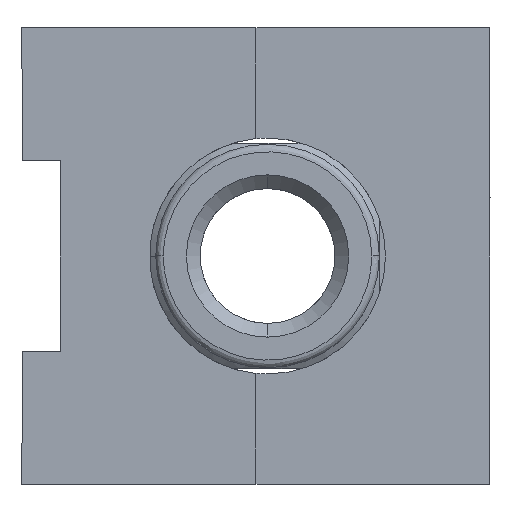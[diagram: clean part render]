
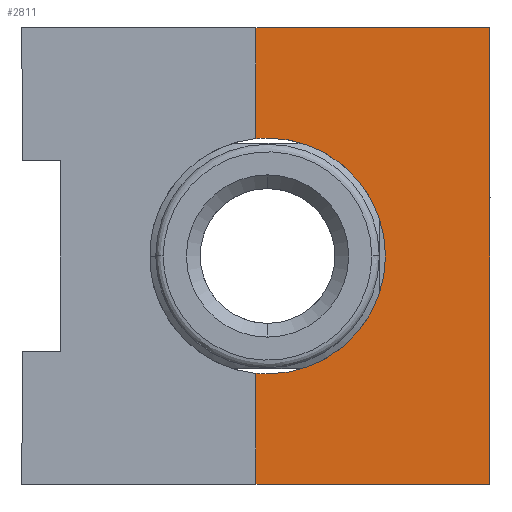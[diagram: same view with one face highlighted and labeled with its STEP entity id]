
A CAD part, left-side view. The second image highlights one B-rep face of the part: STEP entity #2811.
In plain terms, the highlighted planar face has unit normal (-1, 0, 0).
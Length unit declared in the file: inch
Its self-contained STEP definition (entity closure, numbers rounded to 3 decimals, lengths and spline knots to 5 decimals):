
#186 = DIRECTION ( 'NONE',  ( 1., 0., 0. ) ) ;
#281 = CARTESIAN_POINT ( 'NONE',  ( 1.98961, -0.28456, -0.6 ) ) ;
#456 = CIRCLE ( 'NONE', #14050, 0.31 ) ;
#748 = CARTESIAN_POINT ( 'NONE',  ( 1.98961, 0.33044, 0.6 ) ) ;
#859 = ORIENTED_EDGE ( 'NONE', *, *, #3745, .T. ) ;
#975 = CARTESIAN_POINT ( 'NONE',  ( 1.98961, -0.28456, 0.6 ) ) ;
#1020 = CARTESIAN_POINT ( 'NONE',  ( 1.98961, -0.31496, 0. ) ) ;
#1428 = DIRECTION ( 'NONE',  ( 0., 0., -1. ) ) ;
#1697 = VERTEX_POINT ( 'NONE', #14794 ) ;
#1882 = AXIS2_PLACEMENT_3D ( 'NONE', #8262, #4012, #5552 ) ;
#2111 = ORIENTED_EDGE ( 'NONE', *, *, #13435, .T. ) ;
#2472 = VERTEX_POINT ( 'NONE', #7377 ) ;
#2811 = ADVANCED_FACE ( 'NONE', ( #13321 ), #7819, .F. ) ;
#3658 = DIRECTION ( 'NONE',  ( 0., 1., 0. ) ) ;
#3745 = EDGE_CURVE ( 'NONE', #12427, #18177, #10201, .T. ) ;
#4012 = DIRECTION ( 'NONE',  ( 1., 0., 0. ) ) ;
#4221 = LINE ( 'NONE', #975, #6164 ) ;
#4526 = EDGE_CURVE ( 'NONE', #1697, #12427, #4221, .T. ) ;
#4726 = CARTESIAN_POINT ( 'NONE',  ( 1.98961, -0.28456, 0.6 ) ) ;
#5187 = LINE ( 'NONE', #15519, #13426 ) ;
#5552 = DIRECTION ( 'NONE',  ( 0., 0., -1. ) ) ;
#5729 = EDGE_CURVE ( 'NONE', #18177, #12259, #9547, .T. ) ;
#6164 = VECTOR ( 'NONE', #17194, 39.37008 ) ;
#6167 = LINE ( 'NONE', #4726, #6220 ) ;
#6220 = VECTOR ( 'NONE', #14677, 39.37008 ) ;
#7377 = CARTESIAN_POINT ( 'NONE',  ( 1.98961, -0.28456, -0.30851 ) ) ;
#7590 = VECTOR ( 'NONE', #13576, 39.37008 ) ;
#7753 = CARTESIAN_POINT ( 'NONE',  ( 1.98961, -0.31496, 0.31 ) ) ;
#7819 = PLANE ( 'NONE',  #16041 ) ;
#8262 = CARTESIAN_POINT ( 'NONE',  ( 1.98961, -0.31496, 0. ) ) ;
#8572 = CARTESIAN_POINT ( 'NONE',  ( 1.98961, -0.31496, 0. ) ) ;
#8662 = DIRECTION ( 'NONE',  ( 1., 0., 0. ) ) ;
#9135 = CARTESIAN_POINT ( 'NONE',  ( 1.98961, -0.89956, 0.6 ) ) ;
#9434 = DIRECTION ( 'NONE',  ( 0., 0., -1. ) ) ;
#9542 = LINE ( 'NONE', #748, #13119 ) ;
#9547 = CIRCLE ( 'NONE', #15074, 0.31 ) ;
#10201 = CIRCLE ( 'NONE', #1882, 0.31 ) ;
#10587 = LINE ( 'NONE', #9135, #7590 ) ;
#10688 = EDGE_LOOP ( 'NONE', ( #13398, #11957, #859, #17216, #2111, #15624, #19101, #11673 ) ) ;
#11082 = DIRECTION ( 'NONE',  ( 0., -1., 0. ) ) ;
#11673 = ORIENTED_EDGE ( 'NONE', *, *, #16594, .F. ) ;
#11957 = ORIENTED_EDGE ( 'NONE', *, *, #4526, .T. ) ;
#12169 = CARTESIAN_POINT ( 'NONE',  ( 1.98961, -0.89956, 0.6 ) ) ;
#12259 = VERTEX_POINT ( 'NONE', #13588 ) ;
#12387 = EDGE_CURVE ( 'NONE', #12430, #16806, #5187, .T. ) ;
#12427 = VERTEX_POINT ( 'NONE', #15414 ) ;
#12430 = VERTEX_POINT ( 'NONE', #16967 ) ;
#12435 = EDGE_CURVE ( 'NONE', #1697, #15432, #9542, .T. ) ;
#13119 = VECTOR ( 'NONE', #11082, 39.37008 ) ;
#13321 = FACE_OUTER_BOUND ( 'NONE', #10688, .T. ) ;
#13398 = ORIENTED_EDGE ( 'NONE', *, *, #12435, .F. ) ;
#13426 = VECTOR ( 'NONE', #3658, 39.37008 ) ;
#13435 = EDGE_CURVE ( 'NONE', #12259, #2472, #456, .T. ) ;
#13576 = DIRECTION ( 'NONE',  ( 0., 0., -1. ) ) ;
#13588 = CARTESIAN_POINT ( 'NONE',  ( 1.98961, -0.31496, -0.31 ) ) ;
#13874 = DIRECTION ( 'NONE',  ( 1., 0., 0. ) ) ;
#14050 = AXIS2_PLACEMENT_3D ( 'NONE', #1020, #13874, #9434 ) ;
#14677 = DIRECTION ( 'NONE',  ( 0., 0., -1. ) ) ;
#14794 = CARTESIAN_POINT ( 'NONE',  ( 1.98961, -0.28456, 0.6 ) ) ;
#15047 = DIRECTION ( 'NONE',  ( 0., 0., -1. ) ) ;
#15074 = AXIS2_PLACEMENT_3D ( 'NONE', #8572, #8662, #1428 ) ;
#15414 = CARTESIAN_POINT ( 'NONE',  ( 1.98961, -0.28456, 0.30851 ) ) ;
#15432 = VERTEX_POINT ( 'NONE', #12169 ) ;
#15519 = CARTESIAN_POINT ( 'NONE',  ( 1.98961, 0.33044, -0.6 ) ) ;
#15624 = ORIENTED_EDGE ( 'NONE', *, *, #18796, .T. ) ;
#16041 = AXIS2_PLACEMENT_3D ( 'NONE', #16227, #186, #15047 ) ;
#16227 = CARTESIAN_POINT ( 'NONE',  ( 1.98961, 0.33044, 0.6 ) ) ;
#16594 = EDGE_CURVE ( 'NONE', #15432, #12430, #10587, .T. ) ;
#16806 = VERTEX_POINT ( 'NONE', #281 ) ;
#16967 = CARTESIAN_POINT ( 'NONE',  ( 1.98961, -0.89956, -0.6 ) ) ;
#17194 = DIRECTION ( 'NONE',  ( 0., 0., -1. ) ) ;
#17216 = ORIENTED_EDGE ( 'NONE', *, *, #5729, .T. ) ;
#18177 = VERTEX_POINT ( 'NONE', #7753 ) ;
#18796 = EDGE_CURVE ( 'NONE', #2472, #16806, #6167, .T. ) ;
#19101 = ORIENTED_EDGE ( 'NONE', *, *, #12387, .F. ) ;
